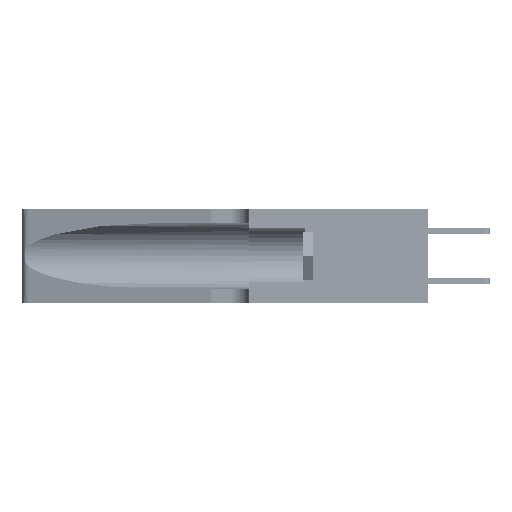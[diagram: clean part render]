
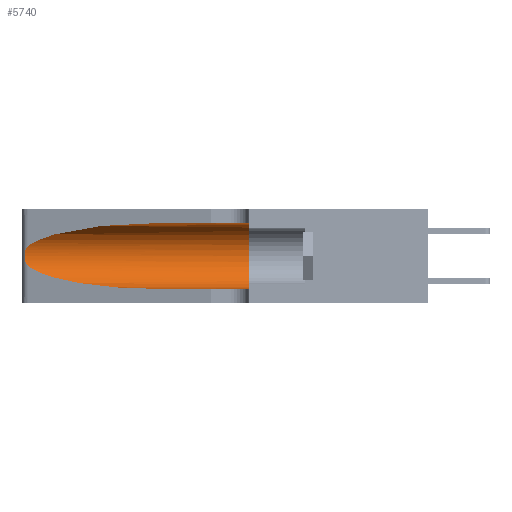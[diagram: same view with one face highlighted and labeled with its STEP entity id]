
A CAD part, left-side view. The second image highlights one B-rep face of the part: STEP entity #5740.
In plain terms, the highlighted cylindrical face has radius 3.308 mm (diameter 6.617 mm), a partial arc.
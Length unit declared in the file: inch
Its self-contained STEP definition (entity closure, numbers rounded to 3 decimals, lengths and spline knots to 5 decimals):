
#217 = CARTESIAN_POINT ( 'NONE',  ( 0.25639, 1.23186, 0.15144 ) ) ;
#701 = ORIENTED_EDGE ( 'NONE', *, *, #33806, .T. ) ;
#1401 = EDGE_LOOP ( 'NONE', ( #26772, #701, #23662, #33646, #30139, #37168 ) ) ;
#2160 = AXIS2_PLACEMENT_3D ( 'NONE', #28396, #16002, #28231 ) ;
#2368 = LINE ( 'NONE', #48706, #44957 ) ;
#2450 = CARTESIAN_POINT ( 'NONE',  ( 0.1305, 0.35, 0.05475 ) ) ;
#2531 = FACE_OUTER_BOUND ( 'NONE', #1401, .T. ) ;
#2844 = CARTESIAN_POINT ( 'NONE',  ( 0.1305, 0.35, 0.185 ) ) ;
#3648 = VERTEX_POINT ( 'NONE', #47609 ) ;
#3972 = VERTEX_POINT ( 'NONE', #8804 ) ;
#4528 = CARTESIAN_POINT ( 'NONE',  ( 0.25787, 1.23484, 0.2124 ) ) ;
#4694 = CARTESIAN_POINT ( 'NONE',  ( 0.25487, 1.22718, 0.14631 ) ) ;
#5438 = CARTESIAN_POINT ( 'NONE',  ( 0.1305, 0.35, 0.31525 ) ) ;
#5740 = ADVANCED_FACE ( 'NONE', ( #2531 ), #45119, .F. ) ;
#6798 = AXIS2_PLACEMENT_3D ( 'NONE', #2844, #11317, #11135 ) ;
#7408 = CARTESIAN_POINT ( 'NONE',  ( 0.25487, 1.22718, 0.22369 ) ) ;
#7790 = B_SPLINE_CURVE_WITH_KNOTS ( 'NONE', 3,
 ( #12146, #49819, #24373, #4528, #28686, #45133, #12498, #41484, #24546, #47922, #8335, #217, #8160, #29225 ),
 .UNSPECIFIED., .F., .F.,
 ( 4, 2, 2, 2, 2, 2, 4 ),
 ( 0., 0.00027, 0.00053, 0.00107, 0.0016, 0.00187, 0.00214 ),
 .UNSPECIFIED. ) ;
#7815 = CARTESIAN_POINT ( 'NONE',  ( 0.1305, 0.72297, 0.31525 ) ) ;
#8160 = CARTESIAN_POINT ( 'NONE',  ( 0.25555, 1.22993, 0.14849 ) ) ;
#8335 = CARTESIAN_POINT ( 'NONE',  ( 0.25789, 1.23486, 0.15765 ) ) ;
#8804 = CARTESIAN_POINT ( 'NONE',  ( 0.25487, 1.22718, 0.22369 ) ) ;
#9066 = VECTOR ( 'NONE', #17888, 39.37008 ) ;
#11135 = DIRECTION ( 'NONE',  ( 0., 0., 1. ) ) ;
#11317 = DIRECTION ( 'NONE',  ( 0., 1., 0. ) ) ;
#11686 = LINE ( 'NONE', #13750, #9066 ) ;
#12146 = CARTESIAN_POINT ( 'NONE',  ( 0.25487, 1.22718, 0.22369 ) ) ;
#12498 = CARTESIAN_POINT ( 'NONE',  ( 0.26075, 1.23896, 0.19203 ) ) ;
#13750 = CARTESIAN_POINT ( 'NONE',  ( 0.1305, 1.61858, 0.31525 ) ) ;
#14998 = CARTESIAN_POINT ( 'NONE',  ( 0.18966, 0.96281, 0.31525 ) ) ;
#16002 = DIRECTION ( 'NONE',  ( 0., -1., 0. ) ) ;
#16134 = EDGE_CURVE ( 'NONE', #40972, #3648, #36519, .T. ) ;
#17171 = CARTESIAN_POINT ( 'NONE',  ( 0.2373, 1.15595, 0.08982 ) ) ;
#17888 = DIRECTION ( 'NONE',  ( 0., -1., 0. ) ) ;
#20939 = CARTESIAN_POINT ( 'NONE',  ( 0.18966, 0.96281, 0.05475 ) ) ;
#21876 = CIRCLE ( 'NONE', #6798, 0.13025 ) ;
#23662 = ORIENTED_EDGE ( 'NONE', *, *, #16134, .T. ) ;
#24373 = CARTESIAN_POINT ( 'NONE',  ( 0.25639, 1.23184, 0.21858 ) ) ;
#24546 = CARTESIAN_POINT ( 'NONE',  ( 0.26017, 1.23833, 0.17102 ) ) ;
#26772 = ORIENTED_EDGE ( 'NONE', *, *, #37695, .T. ) ;
#28231 = DIRECTION ( 'NONE',  ( 0., 0., -1. ) ) ;
#28275 = CARTESIAN_POINT ( 'NONE',  ( 0.25487, 1.22718, 0.14631 ) ) ;
#28396 = CARTESIAN_POINT ( 'NONE',  ( 0.1305, 1.61858, 0.185 ) ) ;
#28686 = CARTESIAN_POINT ( 'NONE',  ( 0.25854, 1.2359, 0.20912 ) ) ;
#29225 = CARTESIAN_POINT ( 'NONE',  ( 0.25487, 1.22718, 0.14631 ) ) ;
#30139 = ORIENTED_EDGE ( 'NONE', *, *, #53395, .F. ) ;
#30651 = CARTESIAN_POINT ( 'NONE',  ( 0.1305, 0.72297, 0.05475 ) ) ;
#31752 = CARTESIAN_POINT ( 'NONE',  ( 0.2373, 1.15595, 0.28018 ) ) ;
#33646 = ORIENTED_EDGE ( 'NONE', *, *, #42943, .T. ) ;
#33806 = EDGE_CURVE ( 'NONE', #3972, #40972, #7790, .T. ) ;
#36519 =( BOUNDED_CURVE ( )  B_SPLINE_CURVE ( 3, ( #4694, #17171, #20939, #30651 ),
 .UNSPECIFIED., .F., .F. ) 
 B_SPLINE_CURVE_WITH_KNOTS ( ( 4, 4 ),
 ( 3.44316, 4.71239 ),
 .UNSPECIFIED. ) 
 CURVE ( )  GEOMETRIC_REPRESENTATION_ITEM ( )  RATIONAL_B_SPLINE_CURVE ( ( 1., 0.87, 0.87, 1. ) ) 
 REPRESENTATION_ITEM ( '' )  );
#37168 = ORIENTED_EDGE ( 'NONE', *, *, #40451, .F. ) ;
#37415 = VERTEX_POINT ( 'NONE', #5438 ) ;
#37695 = EDGE_CURVE ( 'NONE', #49633, #3972, #42152, .T. ) ;
#38908 = VERTEX_POINT ( 'NONE', #2450 ) ;
#40451 = EDGE_CURVE ( 'NONE', #49633, #37415, #11686, .T. ) ;
#40972 = VERTEX_POINT ( 'NONE', #28275 ) ;
#41484 = CARTESIAN_POINT ( 'NONE',  ( 0.26075, 1.23896, 0.178 ) ) ;
#42152 =( BOUNDED_CURVE ( )  B_SPLINE_CURVE ( 3, ( #43501, #14998, #31752, #7408 ),
 .UNSPECIFIED., .F., .T. ) 
 B_SPLINE_CURVE_WITH_KNOTS ( ( 4, 4 ),
 ( 1.5708, 2.84003 ),
 .UNSPECIFIED. ) 
 CURVE ( )  GEOMETRIC_REPRESENTATION_ITEM ( )  RATIONAL_B_SPLINE_CURVE ( ( 1., 0.87, 0.87, 1. ) ) 
 REPRESENTATION_ITEM ( '' )  );
#42943 = EDGE_CURVE ( 'NONE', #3648, #38908, #2368, .T. ) ;
#43501 = CARTESIAN_POINT ( 'NONE',  ( 0.1305, 0.72297, 0.31525 ) ) ;
#44957 = VECTOR ( 'NONE', #53008, 39.37008 ) ;
#45119 = CYLINDRICAL_SURFACE ( 'NONE', #2160, 0.13025 ) ;
#45133 = CARTESIAN_POINT ( 'NONE',  ( 0.26018, 1.23835, 0.19895 ) ) ;
#47609 = CARTESIAN_POINT ( 'NONE',  ( 0.1305, 0.72297, 0.05475 ) ) ;
#47922 = CARTESIAN_POINT ( 'NONE',  ( 0.25856, 1.23593, 0.16098 ) ) ;
#48706 = CARTESIAN_POINT ( 'NONE',  ( 0.1305, 1.61858, 0.05475 ) ) ;
#49633 = VERTEX_POINT ( 'NONE', #7815 ) ;
#49819 = CARTESIAN_POINT ( 'NONE',  ( 0.25555, 1.22994, 0.2215 ) ) ;
#53008 = DIRECTION ( 'NONE',  ( 0., -1., 0. ) ) ;
#53395 = EDGE_CURVE ( 'NONE', #37415, #38908, #21876, .T. ) ;
